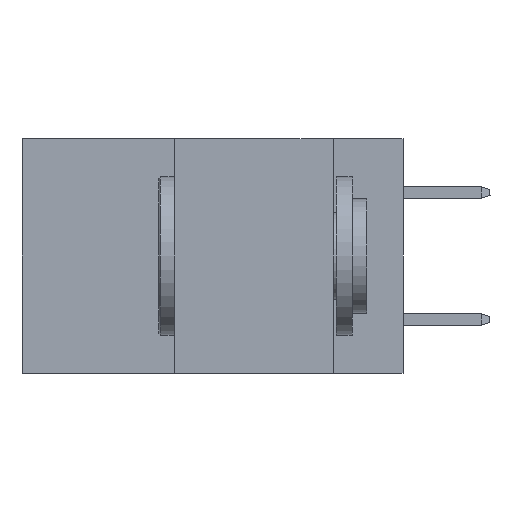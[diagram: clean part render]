
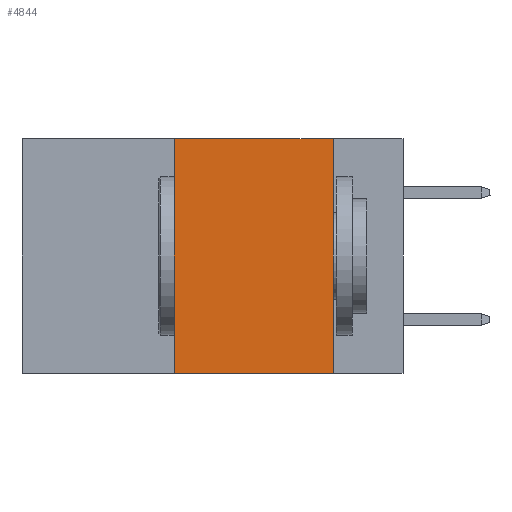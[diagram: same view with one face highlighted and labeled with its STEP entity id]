
A CAD part, left-side view. The second image highlights one B-rep face of the part: STEP entity #4844.
In plain terms, the highlighted planar face has unit normal (-1, 0, 0).
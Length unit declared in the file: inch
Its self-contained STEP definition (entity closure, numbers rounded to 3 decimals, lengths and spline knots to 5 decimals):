
#68 = EDGE_CURVE ( 'NONE', #4933, #11237, #12206, .T. ) ;
#228 = VECTOR ( 'NONE', #2446, 39.37008 ) ;
#256 = DIRECTION ( 'NONE',  ( 0., 0., -1. ) ) ;
#1171 = VERTEX_POINT ( 'NONE', #2967 ) ;
#1478 = DIRECTION ( 'NONE',  ( 0., -1., 0. ) ) ;
#1963 = VECTOR ( 'NONE', #1478, 39.37008 ) ;
#2247 = EDGE_CURVE ( 'NONE', #11237, #1171, #2369, .T. ) ;
#2369 = LINE ( 'NONE', #13237, #228 ) ;
#2446 = DIRECTION ( 'NONE',  ( 0., -1., 0. ) ) ;
#2967 = CARTESIAN_POINT ( 'NONE',  ( 0., 0.11, 0. ) ) ;
#4164 = PLANE ( 'NONE',  #9950 ) ;
#4844 = ADVANCED_FACE ( 'NONE', ( #6842 ), #4164, .F. ) ;
#4906 = VERTEX_POINT ( 'NONE', #16633 ) ;
#4933 = VERTEX_POINT ( 'NONE', #8379 ) ;
#5186 = EDGE_LOOP ( 'NONE', ( #17526, #13182, #12749, #13229 ) ) ;
#5280 = EDGE_CURVE ( 'NONE', #4933, #4906, #16278, .T. ) ;
#5594 = DIRECTION ( 'NONE',  ( 1., 0., 0. ) ) ;
#5873 = VECTOR ( 'NONE', #13711, 39.37008 ) ;
#5984 = DIRECTION ( 'NONE',  ( 0., 0., -1. ) ) ;
#6842 = FACE_OUTER_BOUND ( 'NONE', #5186, .T. ) ;
#7010 = CARTESIAN_POINT ( 'NONE',  ( 0., 0.6, 0. ) ) ;
#7505 = CARTESIAN_POINT ( 'NONE',  ( 0., 0.11, 0. ) ) ;
#8177 = VECTOR ( 'NONE', #5984, 39.37008 ) ;
#8379 = CARTESIAN_POINT ( 'NONE',  ( 0., 0.36, -0.37 ) ) ;
#8381 = CARTESIAN_POINT ( 'NONE',  ( 0., 0.36, 0. ) ) ;
#9697 = CARTESIAN_POINT ( 'NONE',  ( 0., 0.6, -0.37 ) ) ;
#9950 = AXIS2_PLACEMENT_3D ( 'NONE', #7010, #5594, #256 ) ;
#11237 = VERTEX_POINT ( 'NONE', #14608 ) ;
#12206 = LINE ( 'NONE', #8381, #5873 ) ;
#12296 = EDGE_CURVE ( 'NONE', #1171, #4906, #14278, .T. ) ;
#12749 = ORIENTED_EDGE ( 'NONE', *, *, #68, .F. ) ;
#13182 = ORIENTED_EDGE ( 'NONE', *, *, #2247, .F. ) ;
#13229 = ORIENTED_EDGE ( 'NONE', *, *, #5280, .T. ) ;
#13237 = CARTESIAN_POINT ( 'NONE',  ( 0., 0.6, 0. ) ) ;
#13711 = DIRECTION ( 'NONE',  ( 0., 0., 1. ) ) ;
#14278 = LINE ( 'NONE', #7505, #8177 ) ;
#14608 = CARTESIAN_POINT ( 'NONE',  ( 0., 0.36, 0. ) ) ;
#16278 = LINE ( 'NONE', #9697, #1963 ) ;
#16633 = CARTESIAN_POINT ( 'NONE',  ( 0., 0.11, -0.37 ) ) ;
#17526 = ORIENTED_EDGE ( 'NONE', *, *, #12296, .F. ) ;
